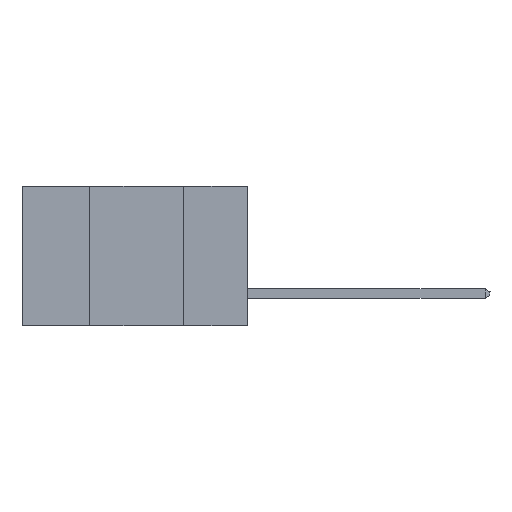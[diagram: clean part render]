
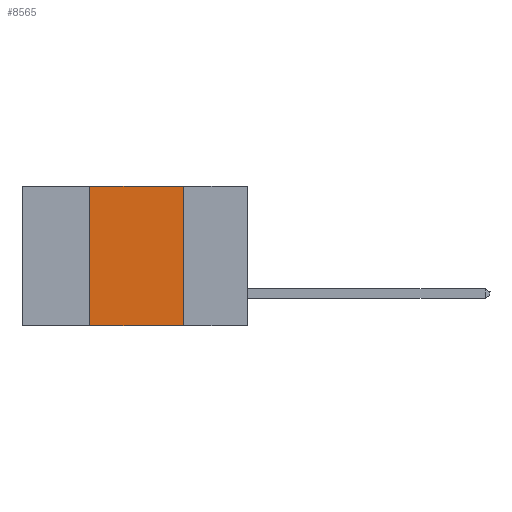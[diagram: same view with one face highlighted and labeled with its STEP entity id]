
A CAD part, left-side view. The second image highlights one B-rep face of the part: STEP entity #8565.
In plain terms, the highlighted planar face has unit normal (-1, 0, 0).
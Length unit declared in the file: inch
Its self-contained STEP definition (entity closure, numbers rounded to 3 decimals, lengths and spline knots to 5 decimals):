
#3 = EDGE_CURVE ( 'NONE', #553, #9447, #3360, .T. ) ;
#553 = VERTEX_POINT ( 'NONE', #10814 ) ;
#1172 = VERTEX_POINT ( 'NONE', #7494 ) ;
#1582 = DIRECTION ( 'NONE',  ( 0., -1., 0. ) ) ;
#1651 = PLANE ( 'NONE',  #11756 ) ;
#3316 = LINE ( 'NONE', #7842, #3930 ) ;
#3360 = LINE ( 'NONE', #8725, #8506 ) ;
#3498 = CARTESIAN_POINT ( 'NONE',  ( 0., 0.42, -0.37 ) ) ;
#3522 = CARTESIAN_POINT ( 'NONE',  ( 0., 0.42, -0.37 ) ) ;
#3639 = CARTESIAN_POINT ( 'NONE',  ( 0., 0.6, 0. ) ) ;
#3702 = DIRECTION ( 'NONE',  ( 0., -1., 0. ) ) ;
#3713 = ORIENTED_EDGE ( 'NONE', *, *, #6337, .F. ) ;
#3930 = VECTOR ( 'NONE', #1582, 39.37008 ) ;
#4166 = EDGE_CURVE ( 'NONE', #1172, #553, #5461, .T. ) ;
#4273 = DIRECTION ( 'NONE',  ( 0., 0., -1. ) ) ;
#5320 = CARTESIAN_POINT ( 'NONE',  ( 0., 0.6, 0. ) ) ;
#5377 = DIRECTION ( 'NONE',  ( 0., 0., 1. ) ) ;
#5461 = LINE ( 'NONE', #3639, #9087 ) ;
#6337 = EDGE_CURVE ( 'NONE', #9331, #1172, #11750, .T. ) ;
#6913 = ORIENTED_EDGE ( 'NONE', *, *, #10827, .T. ) ;
#7182 = DIRECTION ( 'NONE',  ( 0., 0., -1. ) ) ;
#7494 = CARTESIAN_POINT ( 'NONE',  ( 0., 0.42, 0. ) ) ;
#7842 = CARTESIAN_POINT ( 'NONE',  ( 0., 0.6, -0.37 ) ) ;
#8203 = VECTOR ( 'NONE', #5377, 39.37008 ) ;
#8218 = CARTESIAN_POINT ( 'NONE',  ( 0., 0.17, -0.37 ) ) ;
#8506 = VECTOR ( 'NONE', #4273, 39.37008 ) ;
#8565 = ADVANCED_FACE ( 'NONE', ( #9149 ), #1651, .F. ) ;
#8725 = CARTESIAN_POINT ( 'NONE',  ( 0., 0.17, -0.37 ) ) ;
#9087 = VECTOR ( 'NONE', #3702, 39.37008 ) ;
#9149 = FACE_OUTER_BOUND ( 'NONE', #9630, .T. ) ;
#9331 = VERTEX_POINT ( 'NONE', #3522 ) ;
#9447 = VERTEX_POINT ( 'NONE', #8218 ) ;
#9630 = EDGE_LOOP ( 'NONE', ( #10416, #11472, #3713, #6913 ) ) ;
#10048 = DIRECTION ( 'NONE',  ( 1., 0., 0. ) ) ;
#10416 = ORIENTED_EDGE ( 'NONE', *, *, #3, .F. ) ;
#10814 = CARTESIAN_POINT ( 'NONE',  ( 0., 0.17, 0. ) ) ;
#10827 = EDGE_CURVE ( 'NONE', #9331, #9447, #3316, .T. ) ;
#11472 = ORIENTED_EDGE ( 'NONE', *, *, #4166, .F. ) ;
#11750 = LINE ( 'NONE', #3498, #8203 ) ;
#11756 = AXIS2_PLACEMENT_3D ( 'NONE', #5320, #10048, #7182 ) ;
